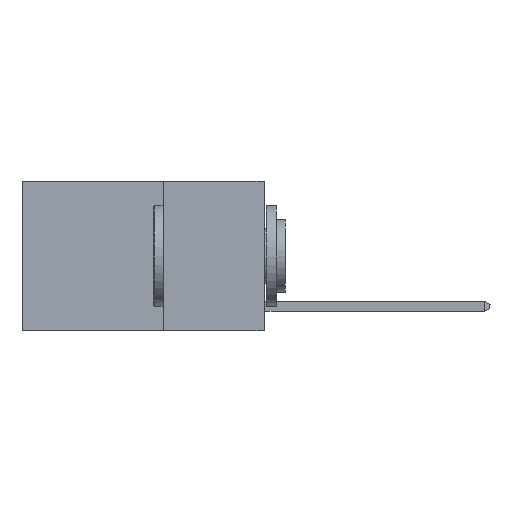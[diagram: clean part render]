
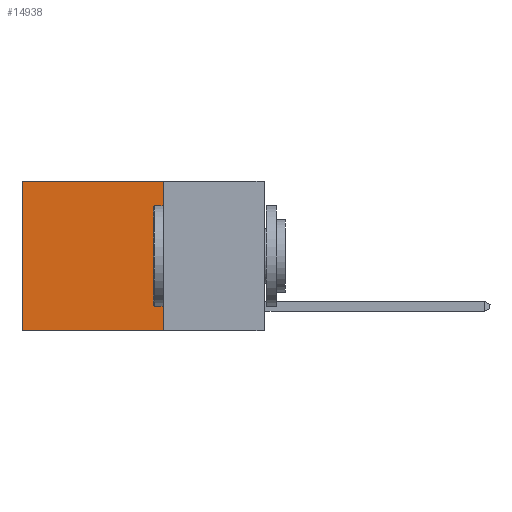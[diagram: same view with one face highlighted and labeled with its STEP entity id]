
A CAD part, left-side view. The second image highlights one B-rep face of the part: STEP entity #14938.
In plain terms, the highlighted planar face has unit normal (-1, 0, 0).
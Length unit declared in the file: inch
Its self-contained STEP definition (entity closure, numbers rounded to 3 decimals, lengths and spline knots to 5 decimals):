
#444 = EDGE_LOOP ( 'NONE', ( #17434, #17866, #16939, #2266 ) ) ;
#1341 = CARTESIAN_POINT ( 'NONE',  ( 0.2625, 0.25, 0. ) ) ;
#2110 = EDGE_CURVE ( 'NONE', #14795, #2582, #5653, .T. ) ;
#2266 = ORIENTED_EDGE ( 'NONE', *, *, #12556, .T. ) ;
#2582 = VERTEX_POINT ( 'NONE', #15749 ) ;
#2715 = PLANE ( 'NONE',  #12939 ) ;
#2911 = DIRECTION ( 'NONE',  ( 0., 0., -1. ) ) ;
#5007 = VECTOR ( 'NONE', #8039, 39.37008 ) ;
#5653 = LINE ( 'NONE', #9606, #12489 ) ;
#5783 = VECTOR ( 'NONE', #2911, 39.37008 ) ;
#6279 = CARTESIAN_POINT ( 'NONE',  ( 0.2625, 0.25, 0. ) ) ;
#6903 = DIRECTION ( 'NONE',  ( 0., 1., 0. ) ) ;
#7311 = DIRECTION ( 'NONE',  ( 0., 0., -1. ) ) ;
#8039 = DIRECTION ( 'NONE',  ( 0., 1., 0. ) ) ;
#8620 = CARTESIAN_POINT ( 'NONE',  ( 0.2625, 0.25, -0.37 ) ) ;
#8720 = EDGE_CURVE ( 'NONE', #18979, #2582, #12758, .T. ) ;
#9312 = LINE ( 'NONE', #17747, #5007 ) ;
#9606 = CARTESIAN_POINT ( 'NONE',  ( 0.2625, 0.6, 0. ) ) ;
#9990 = VECTOR ( 'NONE', #6903, 39.37008 ) ;
#10946 = VERTEX_POINT ( 'NONE', #6279 ) ;
#12364 = EDGE_CURVE ( 'NONE', #10946, #18979, #20230, .T. ) ;
#12489 = VECTOR ( 'NONE', #12773, 39.37008 ) ;
#12556 = EDGE_CURVE ( 'NONE', #10946, #14795, #9312, .T. ) ;
#12758 = LINE ( 'NONE', #13442, #9990 ) ;
#12773 = DIRECTION ( 'NONE',  ( 0., 0., -1. ) ) ;
#12939 = AXIS2_PLACEMENT_3D ( 'NONE', #13935, #17293, #7311 ) ;
#13442 = CARTESIAN_POINT ( 'NONE',  ( 0.2625, 0.25, -0.37 ) ) ;
#13935 = CARTESIAN_POINT ( 'NONE',  ( 0.2625, 0.25, 0. ) ) ;
#14012 = FACE_OUTER_BOUND ( 'NONE', #444, .T. ) ;
#14795 = VERTEX_POINT ( 'NONE', #15054 ) ;
#14938 = ADVANCED_FACE ( 'NONE', ( #14012 ), #2715, .F. ) ;
#15054 = CARTESIAN_POINT ( 'NONE',  ( 0.2625, 0.6, 0. ) ) ;
#15749 = CARTESIAN_POINT ( 'NONE',  ( 0.2625, 0.6, -0.37 ) ) ;
#16939 = ORIENTED_EDGE ( 'NONE', *, *, #12364, .F. ) ;
#17293 = DIRECTION ( 'NONE',  ( 1., 0., 0. ) ) ;
#17434 = ORIENTED_EDGE ( 'NONE', *, *, #2110, .T. ) ;
#17747 = CARTESIAN_POINT ( 'NONE',  ( 0.2625, 0.25, 0. ) ) ;
#17866 = ORIENTED_EDGE ( 'NONE', *, *, #8720, .F. ) ;
#18979 = VERTEX_POINT ( 'NONE', #8620 ) ;
#20230 = LINE ( 'NONE', #1341, #5783 ) ;
